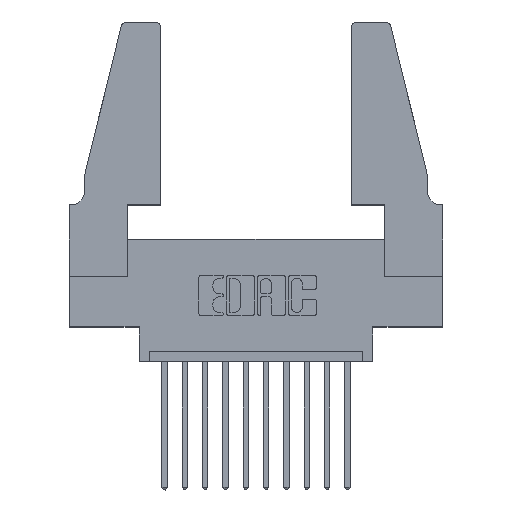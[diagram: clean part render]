
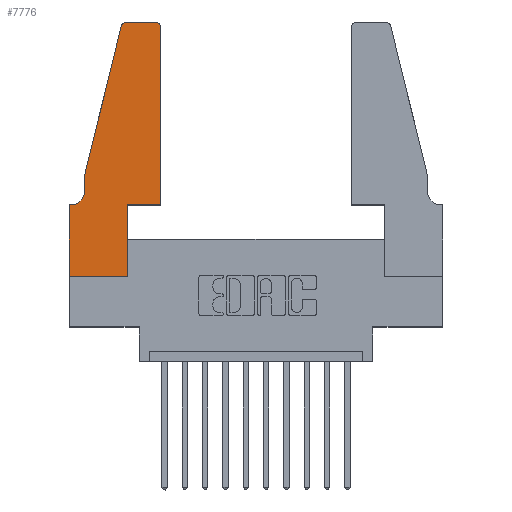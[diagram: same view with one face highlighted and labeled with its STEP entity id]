
A CAD part, top view. The second image highlights one B-rep face of the part: STEP entity #7776.
In plain terms, the highlighted planar face has unit normal (0, 0, 1).
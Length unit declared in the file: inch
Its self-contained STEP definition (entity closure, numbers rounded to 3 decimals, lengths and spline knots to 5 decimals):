
#113 = CARTESIAN_POINT ( 'NONE',  ( 0., 0., 0.37 ) ) ;
#146 = VERTEX_POINT ( 'NONE', #11779 ) ;
#205 = DIRECTION ( 'NONE',  ( 1., 0., 0. ) ) ;
#396 = CARTESIAN_POINT ( 'NONE',  ( 0.0755, 0.5, 0.37 ) ) ;
#411 = CARTESIAN_POINT ( 'NONE',  ( 0.4505, 0.35, 0.37 ) ) ;
#487 = AXIS2_PLACEMENT_3D ( 'NONE', #10577, #11682, #13768 ) ;
#1121 = EDGE_CURVE ( 'NONE', #7227, #9839, #6023, .T. ) ;
#1282 = ORIENTED_EDGE ( 'NONE', *, *, #1981, .T. ) ;
#1533 = VECTOR ( 'NONE', #12525, 39.37008 ) ;
#1543 = VERTEX_POINT ( 'NONE', #12519 ) ;
#1611 = CARTESIAN_POINT ( 'NONE',  ( 0.0755, 0.5, 0.37 ) ) ;
#1669 = ORIENTED_EDGE ( 'NONE', *, *, #7711, .T. ) ;
#1708 = LINE ( 'NONE', #411, #1533 ) ;
#1737 = VECTOR ( 'NONE', #5748, 39.37008 ) ;
#1981 = EDGE_CURVE ( 'NONE', #9099, #10642, #13703, .T. ) ;
#2264 = VECTOR ( 'NONE', #10653, 39.37008 ) ;
#2274 = CARTESIAN_POINT ( 'NONE',  ( 0.0755, 0.35, 0.37 ) ) ;
#2301 = CARTESIAN_POINT ( 'NONE',  ( 0., 0., 0.37 ) ) ;
#2442 = CARTESIAN_POINT ( 'NONE',  ( 0.0055, 0.35, 0.37 ) ) ;
#2703 = DIRECTION ( 'NONE',  ( 1., 0., 0. ) ) ;
#2713 = VECTOR ( 'NONE', #9773, 39.37008 ) ;
#2867 = VERTEX_POINT ( 'NONE', #5680 ) ;
#3257 = VERTEX_POINT ( 'NONE', #5503 ) ;
#3359 = ORIENTED_EDGE ( 'NONE', *, *, #12451, .T. ) ;
#3583 = LINE ( 'NONE', #6447, #2713 ) ;
#3670 = EDGE_CURVE ( 'NONE', #4419, #7227, #3583, .T. ) ;
#3764 = VERTEX_POINT ( 'NONE', #12140 ) ;
#3858 = CARTESIAN_POINT ( 'NONE',  ( 0.2865, 0.35, 0.37 ) ) ;
#4419 = VERTEX_POINT ( 'NONE', #1611 ) ;
#4786 = VECTOR ( 'NONE', #205, 39.37008 ) ;
#4845 = EDGE_CURVE ( 'NONE', #1543, #5596, #11008, .T. ) ;
#4963 = EDGE_CURVE ( 'NONE', #11350, #3764, #13772, .T. ) ;
#5067 = EDGE_CURVE ( 'NONE', #146, #4419, #5090, .T. ) ;
#5090 = LINE ( 'NONE', #396, #11963 ) ;
#5134 = LINE ( 'NONE', #2301, #4786 ) ;
#5503 = CARTESIAN_POINT ( 'NONE',  ( 0.4505, 1.22, 0.37 ) ) ;
#5506 = ORIENTED_EDGE ( 'NONE', *, *, #6842, .T. ) ;
#5596 = VERTEX_POINT ( 'NONE', #3858 ) ;
#5680 = CARTESIAN_POINT ( 'NONE',  ( 0.4505, 0.35, 0.37 ) ) ;
#5748 = DIRECTION ( 'NONE',  ( -1., 0., 0. ) ) ;
#5865 = LINE ( 'NONE', #8395, #2264 ) ;
#5940 = DIRECTION ( 'NONE',  ( -1., 0., 0. ) ) ;
#6023 = CIRCLE ( 'NONE', #11525, 0.07 ) ;
#6033 = CIRCLE ( 'NONE', #487, 0.03 ) ;
#6359 = DIRECTION ( 'NONE',  ( 0., 0., -1. ) ) ;
#6447 = CARTESIAN_POINT ( 'NONE',  ( 0.0755, 0.5, 0.37 ) ) ;
#6515 = ORIENTED_EDGE ( 'NONE', *, *, #5067, .T. ) ;
#6677 = CARTESIAN_POINT ( 'NONE',  ( 0.2605, 1.25, 0.37 ) ) ;
#6687 = EDGE_LOOP ( 'NONE', ( #1282, #8672, #6515, #11477, #8768, #1669, #13596, #11967, #10308, #12052, #3359, #5506 ) ) ;
#6842 = EDGE_CURVE ( 'NONE', #3257, #9099, #11247, .T. ) ;
#7227 = VERTEX_POINT ( 'NONE', #14063 ) ;
#7316 = CARTESIAN_POINT ( 'NONE',  ( 0.4205, 1.25, 0.37 ) ) ;
#7711 = EDGE_CURVE ( 'NONE', #9839, #11350, #10881, .T. ) ;
#7776 = ADVANCED_FACE ( 'NONE', ( #13945 ), #13330, .T. ) ;
#7902 = DIRECTION ( 'NONE',  ( -0.239, -0.971, 0. ) ) ;
#8395 = CARTESIAN_POINT ( 'NONE',  ( 0.4505, 0.35, 0.37 ) ) ;
#8672 = ORIENTED_EDGE ( 'NONE', *, *, #13610, .T. ) ;
#8768 = ORIENTED_EDGE ( 'NONE', *, *, #1121, .T. ) ;
#9099 = VERTEX_POINT ( 'NONE', #7316 ) ;
#9469 = VECTOR ( 'NONE', #11916, 39.37008 ) ;
#9479 = AXIS2_PLACEMENT_3D ( 'NONE', #12529, #12434, #2703 ) ;
#9773 = DIRECTION ( 'NONE',  ( 0., -1., 0. ) ) ;
#9839 = VERTEX_POINT ( 'NONE', #2442 ) ;
#10199 = CARTESIAN_POINT ( 'NONE',  ( 0., 0.35, 0.37 ) ) ;
#10217 = CARTESIAN_POINT ( 'NONE',  ( 0., 0.35, 0.37 ) ) ;
#10308 = ORIENTED_EDGE ( 'NONE', *, *, #4845, .T. ) ;
#10487 = EDGE_CURVE ( 'NONE', #3764, #1543, #5134, .T. ) ;
#10577 = CARTESIAN_POINT ( 'NONE',  ( 0.284, 1.22, 0.37 ) ) ;
#10587 = CARTESIAN_POINT ( 'NONE',  ( 0.0055, 0.42, 0.37 ) ) ;
#10642 = VERTEX_POINT ( 'NONE', #11371 ) ;
#10653 = DIRECTION ( 'NONE',  ( 0., 1., 0. ) ) ;
#10721 = DIRECTION ( 'NONE',  ( -1., 0., 0. ) ) ;
#10859 = DIRECTION ( 'NONE',  ( 0., -1., 0. ) ) ;
#10881 = LINE ( 'NONE', #2274, #12749 ) ;
#11008 = LINE ( 'NONE', #13911, #9469 ) ;
#11020 = EDGE_CURVE ( 'NONE', #5596, #2867, #1708, .T. ) ;
#11107 = VECTOR ( 'NONE', #10859, 39.37008 ) ;
#11247 = CIRCLE ( 'NONE', #9479, 0.03 ) ;
#11350 = VERTEX_POINT ( 'NONE', #10199 ) ;
#11371 = CARTESIAN_POINT ( 'NONE',  ( 0.284, 1.25, 0.37 ) ) ;
#11477 = ORIENTED_EDGE ( 'NONE', *, *, #3670, .T. ) ;
#11525 = AXIS2_PLACEMENT_3D ( 'NONE', #10587, #6359, #10721 ) ;
#11682 = DIRECTION ( 'NONE',  ( 0., 0., 1. ) ) ;
#11779 = CARTESIAN_POINT ( 'NONE',  ( 0.25487, 1.22718, 0.37 ) ) ;
#11916 = DIRECTION ( 'NONE',  ( 0., 1., 0. ) ) ;
#11963 = VECTOR ( 'NONE', #7902, 39.37008 ) ;
#11967 = ORIENTED_EDGE ( 'NONE', *, *, #10487, .T. ) ;
#12052 = ORIENTED_EDGE ( 'NONE', *, *, #11020, .T. ) ;
#12140 = CARTESIAN_POINT ( 'NONE',  ( 0., 0., 0.37 ) ) ;
#12316 = AXIS2_PLACEMENT_3D ( 'NONE', #10217, #12409, #13509 ) ;
#12409 = DIRECTION ( 'NONE',  ( 0., 0., 1. ) ) ;
#12434 = DIRECTION ( 'NONE',  ( 0., 0., 1. ) ) ;
#12451 = EDGE_CURVE ( 'NONE', #2867, #3257, #5865, .T. ) ;
#12519 = CARTESIAN_POINT ( 'NONE',  ( 0.2865, 0., 0.37 ) ) ;
#12525 = DIRECTION ( 'NONE',  ( 1., 0., 0. ) ) ;
#12529 = CARTESIAN_POINT ( 'NONE',  ( 0.4205, 1.22, 0.37 ) ) ;
#12749 = VECTOR ( 'NONE', #5940, 39.37008 ) ;
#13330 = PLANE ( 'NONE',  #12316 ) ;
#13509 = DIRECTION ( 'NONE',  ( 1., 0., 0. ) ) ;
#13596 = ORIENTED_EDGE ( 'NONE', *, *, #4963, .T. ) ;
#13610 = EDGE_CURVE ( 'NONE', #10642, #146, #6033, .T. ) ;
#13703 = LINE ( 'NONE', #6677, #1737 ) ;
#13768 = DIRECTION ( 'NONE',  ( 1., 0., 0. ) ) ;
#13772 = LINE ( 'NONE', #113, #11107 ) ;
#13911 = CARTESIAN_POINT ( 'NONE',  ( 0.2865, 0.35, 0.37 ) ) ;
#13945 = FACE_OUTER_BOUND ( 'NONE', #6687, .T. ) ;
#14063 = CARTESIAN_POINT ( 'NONE',  ( 0.0755, 0.42, 0.37 ) ) ;
